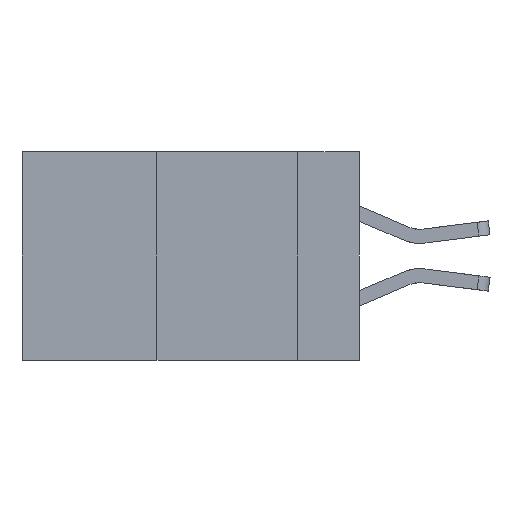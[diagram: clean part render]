
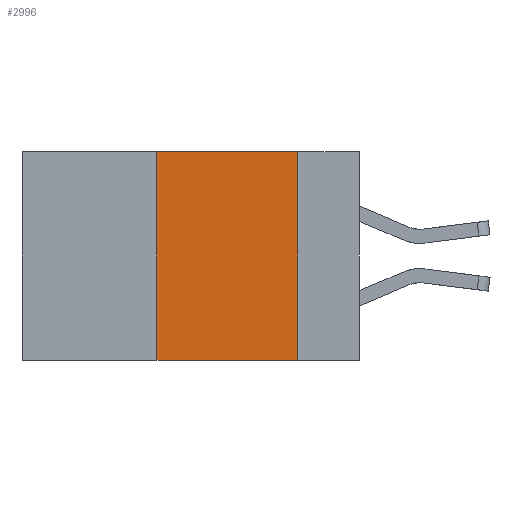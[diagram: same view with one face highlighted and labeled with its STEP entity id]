
A CAD part, left-side view. The second image highlights one B-rep face of the part: STEP entity #2996.
In plain terms, the highlighted planar face has unit normal (-1, 0, 0).
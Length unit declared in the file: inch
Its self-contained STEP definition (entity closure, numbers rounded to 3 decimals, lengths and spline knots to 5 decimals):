
#1374 = LINE ( 'NONE', #6996, #6669 ) ;
#1761 = DIRECTION ( 'NONE',  ( 0., 0., 1. ) ) ;
#2693 = CARTESIAN_POINT ( 'NONE',  ( 0., 0.6, 0. ) ) ;
#2737 = EDGE_CURVE ( 'NONE', #6516, #4801, #1374, .T. ) ;
#2996 = ADVANCED_FACE ( 'NONE', ( #8828 ), #11222, .F. ) ;
#3155 = CARTESIAN_POINT ( 'NONE',  ( 0., 0.36, 0. ) ) ;
#3187 = ORIENTED_EDGE ( 'NONE', *, *, #7930, .F. ) ;
#3855 = CARTESIAN_POINT ( 'NONE',  ( 0., 0.11, -0.37 ) ) ;
#4801 = VERTEX_POINT ( 'NONE', #3155 ) ;
#5371 = EDGE_CURVE ( 'NONE', #6516, #7387, #5656, .T. ) ;
#5656 = LINE ( 'NONE', #6062, #8013 ) ;
#5966 = ORIENTED_EDGE ( 'NONE', *, *, #2737, .F. ) ;
#6062 = CARTESIAN_POINT ( 'NONE',  ( 0., 0.6, -0.37 ) ) ;
#6387 = CARTESIAN_POINT ( 'NONE',  ( 0., 0.6, 0. ) ) ;
#6516 = VERTEX_POINT ( 'NONE', #7649 ) ;
#6554 = LINE ( 'NONE', #2693, #6857 ) ;
#6669 = VECTOR ( 'NONE', #1761, 39.37008 ) ;
#6682 = CARTESIAN_POINT ( 'NONE',  ( 0., 0.11, 0. ) ) ;
#6857 = VECTOR ( 'NONE', #8809, 39.37008 ) ;
#6996 = CARTESIAN_POINT ( 'NONE',  ( 0., 0.36, 0. ) ) ;
#7175 = AXIS2_PLACEMENT_3D ( 'NONE', #6387, #13134, #7388 ) ;
#7387 = VERTEX_POINT ( 'NONE', #3855 ) ;
#7388 = DIRECTION ( 'NONE',  ( 0., 0., -1. ) ) ;
#7649 = CARTESIAN_POINT ( 'NONE',  ( 0., 0.36, -0.37 ) ) ;
#7679 = EDGE_LOOP ( 'NONE', ( #10836, #3187, #5966, #11149 ) ) ;
#7930 = EDGE_CURVE ( 'NONE', #4801, #12867, #6554, .T. ) ;
#8013 = VECTOR ( 'NONE', #11909, 39.37008 ) ;
#8633 = CARTESIAN_POINT ( 'NONE',  ( 0., 0.11, 0. ) ) ;
#8809 = DIRECTION ( 'NONE',  ( 0., -1., 0. ) ) ;
#8828 = FACE_OUTER_BOUND ( 'NONE', #7679, .T. ) ;
#10249 = EDGE_CURVE ( 'NONE', #12867, #7387, #10298, .T. ) ;
#10298 = LINE ( 'NONE', #6682, #12843 ) ;
#10836 = ORIENTED_EDGE ( 'NONE', *, *, #10249, .F. ) ;
#11149 = ORIENTED_EDGE ( 'NONE', *, *, #5371, .T. ) ;
#11222 = PLANE ( 'NONE',  #7175 ) ;
#11909 = DIRECTION ( 'NONE',  ( 0., -1., 0. ) ) ;
#12461 = DIRECTION ( 'NONE',  ( 0., 0., -1. ) ) ;
#12843 = VECTOR ( 'NONE', #12461, 39.37008 ) ;
#12867 = VERTEX_POINT ( 'NONE', #8633 ) ;
#13134 = DIRECTION ( 'NONE',  ( 1., 0., 0. ) ) ;
